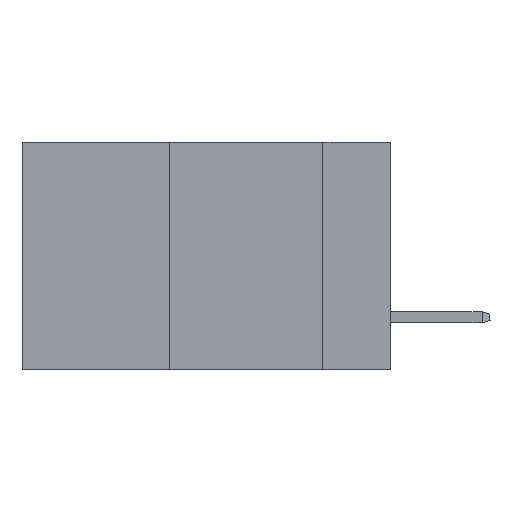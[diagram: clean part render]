
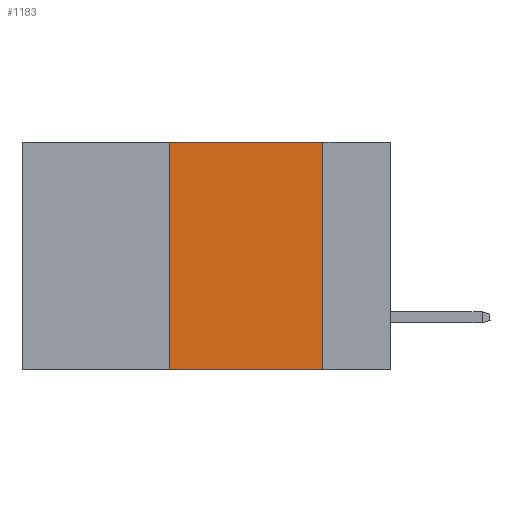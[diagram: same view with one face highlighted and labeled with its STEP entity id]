
A CAD part, left-side view. The second image highlights one B-rep face of the part: STEP entity #1183.
In plain terms, the highlighted planar face has unit normal (-1, 0, 0).
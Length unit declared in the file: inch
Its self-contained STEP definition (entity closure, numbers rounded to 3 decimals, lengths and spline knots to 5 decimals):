
#319 = CARTESIAN_POINT ( 'NONE',  ( 0., 0.6, -0.37 ) ) ;
#547 = ORIENTED_EDGE ( 'NONE', *, *, #5428, .T. ) ;
#662 = EDGE_CURVE ( 'NONE', #9198, #11286, #5079, .T. ) ;
#965 = DIRECTION ( 'NONE',  ( 1., 0., 0. ) ) ;
#1183 = ADVANCED_FACE ( 'NONE', ( #16368 ), #10925, .F. ) ;
#2246 = CARTESIAN_POINT ( 'NONE',  ( 0., 0.6, 0. ) ) ;
#2848 = CARTESIAN_POINT ( 'NONE',  ( 0., 0.36, 0. ) ) ;
#3399 = DIRECTION ( 'NONE',  ( 0., -1., 0. ) ) ;
#3955 = LINE ( 'NONE', #319, #10750 ) ;
#4105 = ORIENTED_EDGE ( 'NONE', *, *, #13967, .F. ) ;
#4391 = LINE ( 'NONE', #12532, #7315 ) ;
#5079 = LINE ( 'NONE', #9234, #10933 ) ;
#5428 = EDGE_CURVE ( 'NONE', #7797, #17902, #3955, .T. ) ;
#5777 = EDGE_CURVE ( 'NONE', #11286, #17902, #4391, .T. ) ;
#7315 = VECTOR ( 'NONE', #15461, 39.37008 ) ;
#7603 = CARTESIAN_POINT ( 'NONE',  ( 0., 0.11, 0. ) ) ;
#7797 = VERTEX_POINT ( 'NONE', #18544 ) ;
#8872 = VECTOR ( 'NONE', #15644, 39.37008 ) ;
#8873 = DIRECTION ( 'NONE',  ( 0., -1., 0. ) ) ;
#9198 = VERTEX_POINT ( 'NONE', #11397 ) ;
#9234 = CARTESIAN_POINT ( 'NONE',  ( 0., 0.6, 0. ) ) ;
#10750 = VECTOR ( 'NONE', #8873, 39.37008 ) ;
#10925 = PLANE ( 'NONE',  #11877 ) ;
#10933 = VECTOR ( 'NONE', #3399, 39.37008 ) ;
#11143 = EDGE_LOOP ( 'NONE', ( #16598, #14176, #4105, #547 ) ) ;
#11286 = VERTEX_POINT ( 'NONE', #7603 ) ;
#11397 = CARTESIAN_POINT ( 'NONE',  ( 0., 0.36, 0. ) ) ;
#11877 = AXIS2_PLACEMENT_3D ( 'NONE', #2246, #965, #18367 ) ;
#12532 = CARTESIAN_POINT ( 'NONE',  ( 0., 0.11, 0. ) ) ;
#12695 = LINE ( 'NONE', #2848, #8872 ) ;
#13967 = EDGE_CURVE ( 'NONE', #7797, #9198, #12695, .T. ) ;
#14176 = ORIENTED_EDGE ( 'NONE', *, *, #662, .F. ) ;
#15461 = DIRECTION ( 'NONE',  ( 0., 0., -1. ) ) ;
#15644 = DIRECTION ( 'NONE',  ( 0., 0., 1. ) ) ;
#16368 = FACE_OUTER_BOUND ( 'NONE', #11143, .T. ) ;
#16598 = ORIENTED_EDGE ( 'NONE', *, *, #5777, .F. ) ;
#17802 = CARTESIAN_POINT ( 'NONE',  ( 0., 0.11, -0.37 ) ) ;
#17902 = VERTEX_POINT ( 'NONE', #17802 ) ;
#18367 = DIRECTION ( 'NONE',  ( 0., 0., -1. ) ) ;
#18544 = CARTESIAN_POINT ( 'NONE',  ( 0., 0.36, -0.37 ) ) ;
